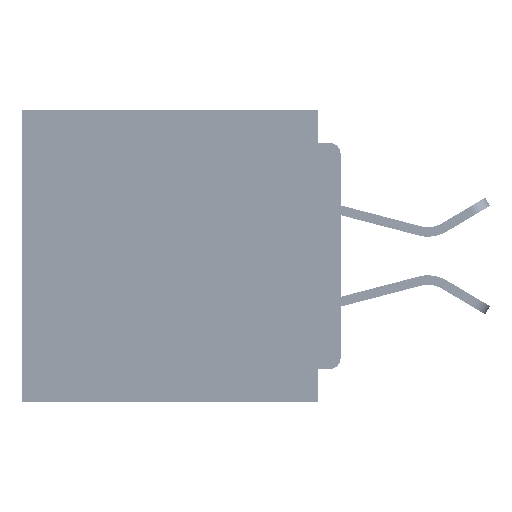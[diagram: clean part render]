
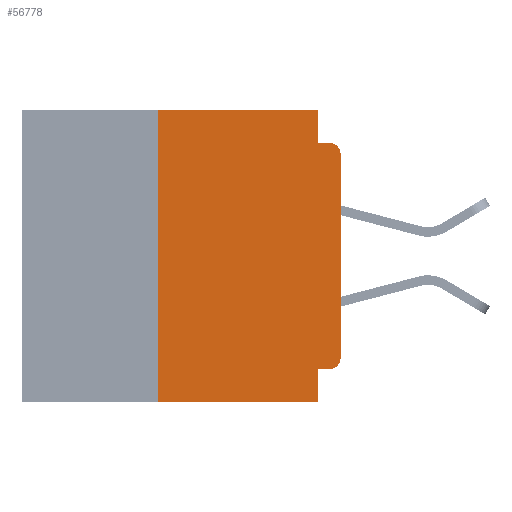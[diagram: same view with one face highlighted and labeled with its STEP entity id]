
A CAD part, left-side view. The second image highlights one B-rep face of the part: STEP entity #56778.
In plain terms, the highlighted planar face has unit normal (-1, 0, 0).
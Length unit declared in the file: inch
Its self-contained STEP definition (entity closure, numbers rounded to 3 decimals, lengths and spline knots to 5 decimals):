
#125 = DIRECTION ( 'NONE',  ( 0., -1., 0. ) ) ;
#1534 = CARTESIAN_POINT ( 'NONE',  ( 0., 0., -0.045 ) ) ;
#2470 = CARTESIAN_POINT ( 'NONE',  ( 0., 0.015, -0.06 ) ) ;
#3371 = VERTEX_POINT ( 'NONE', #35217 ) ;
#3681 = EDGE_CURVE ( 'NONE', #3371, #35581, #25087, .T. ) ;
#4190 = LINE ( 'NONE', #29234, #47477 ) ;
#5999 = ORIENTED_EDGE ( 'NONE', *, *, #48826, .F. ) ;
#7022 = DIRECTION ( 'NONE',  ( 0., 0., -1. ) ) ;
#7327 = CARTESIAN_POINT ( 'NONE',  ( 0., 0., 0. ) ) ;
#7468 = EDGE_CURVE ( 'NONE', #54442, #33077, #18248, .T. ) ;
#7832 = DIRECTION ( 'NONE',  ( 0., -1., 0. ) ) ;
#8733 = CARTESIAN_POINT ( 'NONE',  ( 0., 0.031, 0. ) ) ;
#8746 = EDGE_CURVE ( 'NONE', #10938, #30504, #19490, .T. ) ;
#8799 = CARTESIAN_POINT ( 'NONE',  ( 0., 0.031, -0.4 ) ) ;
#9805 = CARTESIAN_POINT ( 'NONE',  ( 0., 0.015, -0.045 ) ) ;
#10717 = LINE ( 'NONE', #8799, #43562 ) ;
#10812 = CARTESIAN_POINT ( 'NONE',  ( 0., 0.015, -0.34 ) ) ;
#10938 = VERTEX_POINT ( 'NONE', #24362 ) ;
#12007 = CARTESIAN_POINT ( 'NONE',  ( 0., 0.25, -0.4 ) ) ;
#12432 = VERTEX_POINT ( 'NONE', #54997 ) ;
#14342 = CIRCLE ( 'NONE', #36119, 0.015 ) ;
#15223 = CARTESIAN_POINT ( 'NONE',  ( 0., 0.25, -0.4 ) ) ;
#15306 = DIRECTION ( 'NONE',  ( 0., 0., -1. ) ) ;
#15411 = DIRECTION ( 'NONE',  ( 0., 0., 1. ) ) ;
#15738 = PLANE ( 'NONE',  #52056 ) ;
#16481 = CARTESIAN_POINT ( 'NONE',  ( 0., 0.031, -0.4 ) ) ;
#18248 = LINE ( 'NONE', #31472, #28810 ) ;
#18641 = ORIENTED_EDGE ( 'NONE', *, *, #3681, .T. ) ;
#19292 = EDGE_CURVE ( 'NONE', #51827, #52543, #14342, .T. ) ;
#19452 = LINE ( 'NONE', #7327, #43221 ) ;
#19490 = LINE ( 'NONE', #8733, #30048 ) ;
#19927 = ORIENTED_EDGE ( 'NONE', *, *, #57626, .F. ) ;
#20245 = CARTESIAN_POINT ( 'NONE',  ( 0., 0.437, 0. ) ) ;
#20813 = DIRECTION ( 'NONE',  ( 0., 0., 1. ) ) ;
#22032 = DIRECTION ( 'NONE',  ( 0., 0., -1. ) ) ;
#22772 = LINE ( 'NONE', #52674, #46493 ) ;
#24362 = CARTESIAN_POINT ( 'NONE',  ( 0., 0.031, 0. ) ) ;
#25087 = CIRCLE ( 'NONE', #30884, 0.015 ) ;
#28387 = ORIENTED_EDGE ( 'NONE', *, *, #28615, .F. ) ;
#28615 = EDGE_CURVE ( 'NONE', #51827, #47337, #4190, .T. ) ;
#28810 = VECTOR ( 'NONE', #125, 39.37008 ) ;
#29234 = CARTESIAN_POINT ( 'NONE',  ( 0., 0., -0.355 ) ) ;
#29295 = DIRECTION ( 'NONE',  ( 0., 0., -1. ) ) ;
#29955 = LINE ( 'NONE', #15223, #40381 ) ;
#30043 = CARTESIAN_POINT ( 'NONE',  ( 0., 0., -0.34 ) ) ;
#30048 = VECTOR ( 'NONE', #22032, 39.37008 ) ;
#30504 = VERTEX_POINT ( 'NONE', #34014 ) ;
#30856 = ORIENTED_EDGE ( 'NONE', *, *, #8746, .F. ) ;
#30884 = AXIS2_PLACEMENT_3D ( 'NONE', #2470, #33839, #7022 ) ;
#31472 = CARTESIAN_POINT ( 'NONE',  ( 0., 0.437, -0.4 ) ) ;
#31732 = EDGE_CURVE ( 'NONE', #12432, #10938, #22772, .T. ) ;
#33077 = VERTEX_POINT ( 'NONE', #16481 ) ;
#33839 = DIRECTION ( 'NONE',  ( -1., 0., 0. ) ) ;
#34014 = CARTESIAN_POINT ( 'NONE',  ( 0., 0.031, -0.045 ) ) ;
#34092 = ORIENTED_EDGE ( 'NONE', *, *, #39729, .F. ) ;
#35217 = CARTESIAN_POINT ( 'NONE',  ( 0., 0., -0.06 ) ) ;
#35376 = ORIENTED_EDGE ( 'NONE', *, *, #31732, .F. ) ;
#35581 = VERTEX_POINT ( 'NONE', #9805 ) ;
#36119 = AXIS2_PLACEMENT_3D ( 'NONE', #10812, #42054, #15306 ) ;
#36538 = ORIENTED_EDGE ( 'NONE', *, *, #7468, .T. ) ;
#37071 = CARTESIAN_POINT ( 'NONE',  ( 0., 0.015, -0.355 ) ) ;
#39729 = EDGE_CURVE ( 'NONE', #30504, #35581, #44578, .T. ) ;
#40381 = VECTOR ( 'NONE', #15411, 39.37008 ) ;
#40727 = EDGE_LOOP ( 'NONE', ( #42070, #18641, #34092, #30856, #35376, #5999, #36538, #19927, #28387, #54306 ) ) ;
#42054 = DIRECTION ( 'NONE',  ( -1., 0., 0. ) ) ;
#42070 = ORIENTED_EDGE ( 'NONE', *, *, #47701, .T. ) ;
#43221 = VECTOR ( 'NONE', #20813, 39.37008 ) ;
#43562 = VECTOR ( 'NONE', #44547, 39.37008 ) ;
#44076 = CARTESIAN_POINT ( 'NONE',  ( 0., 0.031, -0.355 ) ) ;
#44547 = DIRECTION ( 'NONE',  ( 0., 0., -1. ) ) ;
#44578 = LINE ( 'NONE', #1534, #53581 ) ;
#46493 = VECTOR ( 'NONE', #7832, 39.37008 ) ;
#47337 = VERTEX_POINT ( 'NONE', #44076 ) ;
#47477 = VECTOR ( 'NONE', #51539, 39.37008 ) ;
#47701 = EDGE_CURVE ( 'NONE', #52543, #3371, #19452, .T. ) ;
#48826 = EDGE_CURVE ( 'NONE', #54442, #12432, #29955, .T. ) ;
#51539 = DIRECTION ( 'NONE',  ( 0., 1., 0. ) ) ;
#51827 = VERTEX_POINT ( 'NONE', #37071 ) ;
#52056 = AXIS2_PLACEMENT_3D ( 'NONE', #20245, #55851, #29295 ) ;
#52543 = VERTEX_POINT ( 'NONE', #30043 ) ;
#52674 = CARTESIAN_POINT ( 'NONE',  ( 0., 0.437, 0. ) ) ;
#53581 = VECTOR ( 'NONE', #54995, 39.37008 ) ;
#54306 = ORIENTED_EDGE ( 'NONE', *, *, #19292, .T. ) ;
#54442 = VERTEX_POINT ( 'NONE', #12007 ) ;
#54995 = DIRECTION ( 'NONE',  ( 0., -1., 0. ) ) ;
#54997 = CARTESIAN_POINT ( 'NONE',  ( 0., 0.25, 0. ) ) ;
#55851 = DIRECTION ( 'NONE',  ( 1., 0., 0. ) ) ;
#56778 = ADVANCED_FACE ( 'NONE', ( #56826 ), #15738, .F. ) ;
#56826 = FACE_OUTER_BOUND ( 'NONE', #40727, .T. ) ;
#57626 = EDGE_CURVE ( 'NONE', #47337, #33077, #10717, .T. ) ;
